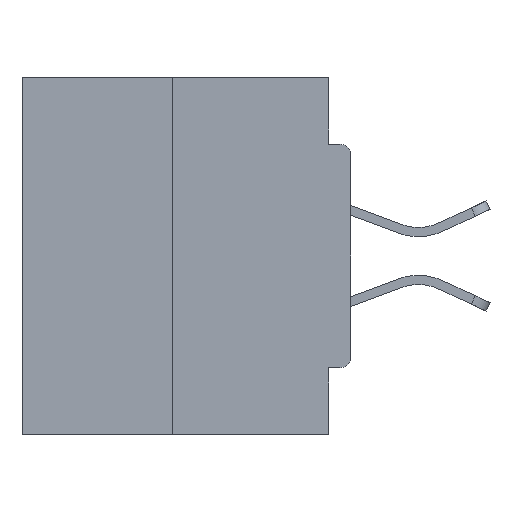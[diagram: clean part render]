
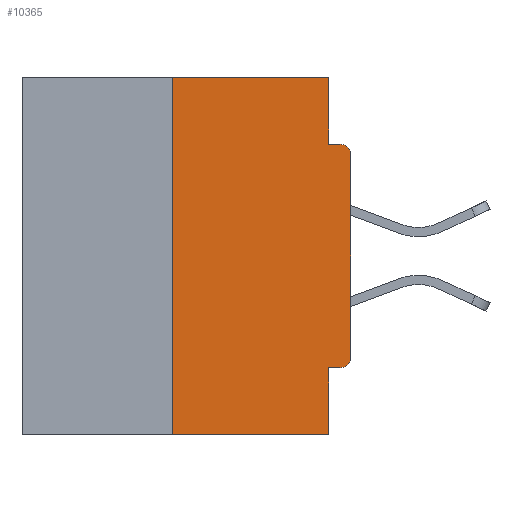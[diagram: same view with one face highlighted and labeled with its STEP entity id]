
A CAD part, left-side view. The second image highlights one B-rep face of the part: STEP entity #10365.
In plain terms, the highlighted planar face has unit normal (-1, 0, 0).
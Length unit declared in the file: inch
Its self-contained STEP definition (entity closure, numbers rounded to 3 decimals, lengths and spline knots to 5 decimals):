
#376 = VECTOR ( 'NONE', #6694, 39.37008 ) ;
#420 = CARTESIAN_POINT ( 'NONE',  ( 0., 0.031, -0.5 ) ) ;
#724 = CARTESIAN_POINT ( 'NONE',  ( 0., 0.031, 0. ) ) ;
#1459 = LINE ( 'NONE', #4553, #17671 ) ;
#1939 = AXIS2_PLACEMENT_3D ( 'NONE', #21516, #30189, #21997 ) ;
#2133 = ORIENTED_EDGE ( 'NONE', *, *, #30267, .T. ) ;
#2251 = EDGE_LOOP ( 'NONE', ( #25524, #4709, #2133, #23375, #24445, #21323, #34818, #24912, #11728, #12745 ) ) ;
#2271 = VECTOR ( 'NONE', #32624, 39.37008 ) ;
#2527 = LINE ( 'NONE', #28972, #376 ) ;
#2691 = LINE ( 'NONE', #9984, #2271 ) ;
#3945 = DIRECTION ( 'NONE',  ( 0., 0., -1. ) ) ;
#4428 = LINE ( 'NONE', #32149, #32079 ) ;
#4553 = CARTESIAN_POINT ( 'NONE',  ( 0., 0.46, 0. ) ) ;
#4709 = ORIENTED_EDGE ( 'NONE', *, *, #26231, .F. ) ;
#4724 = LINE ( 'NONE', #21037, #30146 ) ;
#4948 = PLANE ( 'NONE',  #1939 ) ;
#5551 = EDGE_CURVE ( 'NONE', #19096, #10292, #28142, .T. ) ;
#6506 = CARTESIAN_POINT ( 'NONE',  ( 0., 0.015, -0.4065 ) ) ;
#6694 = DIRECTION ( 'NONE',  ( 0., -1., 0. ) ) ;
#6846 = VERTEX_POINT ( 'NONE', #6506 ) ;
#8328 = VERTEX_POINT ( 'NONE', #724 ) ;
#9816 = CARTESIAN_POINT ( 'NONE',  ( 0., 0.031, -0.4065 ) ) ;
#9984 = CARTESIAN_POINT ( 'NONE',  ( 0., 0.031, -0.5 ) ) ;
#10292 = VERTEX_POINT ( 'NONE', #31576 ) ;
#10296 = CARTESIAN_POINT ( 'NONE',  ( 0., 0., -0.0935 ) ) ;
#10365 = ADVANCED_FACE ( 'NONE', ( #22548 ), #4948, .F. ) ;
#11728 = ORIENTED_EDGE ( 'NONE', *, *, #5551, .F. ) ;
#12745 = ORIENTED_EDGE ( 'NONE', *, *, #33685, .F. ) ;
#13715 = LINE ( 'NONE', #23313, #28602 ) ;
#13909 = VERTEX_POINT ( 'NONE', #420 ) ;
#14108 = CARTESIAN_POINT ( 'NONE',  ( 0., 0., -0.3915 ) ) ;
#15509 = CARTESIAN_POINT ( 'NONE',  ( 0., 0., -0.1085 ) ) ;
#15865 = VERTEX_POINT ( 'NONE', #9816 ) ;
#17099 = CIRCLE ( 'NONE', #17959, 0.015 ) ;
#17471 = CARTESIAN_POINT ( 'NONE',  ( 0., 0., -0.4065 ) ) ;
#17671 = VECTOR ( 'NONE', #32504, 39.37008 ) ;
#17777 = VERTEX_POINT ( 'NONE', #14108 ) ;
#17883 = CARTESIAN_POINT ( 'NONE',  ( 0., 0.25, 0. ) ) ;
#17959 = AXIS2_PLACEMENT_3D ( 'NONE', #34139, #26524, #26048 ) ;
#18327 = DIRECTION ( 'NONE',  ( 0., 0., 1. ) ) ;
#18349 = EDGE_CURVE ( 'NONE', #6846, #15865, #21427, .T. ) ;
#19096 = VERTEX_POINT ( 'NONE', #30796 ) ;
#19836 = VERTEX_POINT ( 'NONE', #20727 ) ;
#20727 = CARTESIAN_POINT ( 'NONE',  ( 0., 0.25, -0.5 ) ) ;
#20875 = CARTESIAN_POINT ( 'NONE',  ( 0., 0.015, -0.3915 ) ) ;
#21037 = CARTESIAN_POINT ( 'NONE',  ( 0., 0., 0. ) ) ;
#21323 = ORIENTED_EDGE ( 'NONE', *, *, #22582, .T. ) ;
#21427 = LINE ( 'NONE', #17471, #28906 ) ;
#21516 = CARTESIAN_POINT ( 'NONE',  ( 0., 0.46, 0. ) ) ;
#21997 = DIRECTION ( 'NONE',  ( 0., 0., -1. ) ) ;
#22548 = FACE_OUTER_BOUND ( 'NONE', #2251, .T. ) ;
#22582 = EDGE_CURVE ( 'NONE', #6846, #17777, #36241, .T. ) ;
#22743 = DIRECTION ( 'NONE',  ( 0., 1., 0. ) ) ;
#23313 = CARTESIAN_POINT ( 'NONE',  ( 0., 0.031, 0. ) ) ;
#23375 = ORIENTED_EDGE ( 'NONE', *, *, #35879, .F. ) ;
#24173 = DIRECTION ( 'NONE',  ( 0., 0., 1. ) ) ;
#24445 = ORIENTED_EDGE ( 'NONE', *, *, #18349, .F. ) ;
#24912 = ORIENTED_EDGE ( 'NONE', *, *, #34649, .T. ) ;
#25524 = ORIENTED_EDGE ( 'NONE', *, *, #33356, .F. ) ;
#25990 = VECTOR ( 'NONE', #35535, 39.37008 ) ;
#26048 = DIRECTION ( 'NONE',  ( 0., 0., -1. ) ) ;
#26112 = DIRECTION ( 'NONE',  ( 0., 0., -1. ) ) ;
#26231 = EDGE_CURVE ( 'NONE', #19836, #28730, #4428, .T. ) ;
#26524 = DIRECTION ( 'NONE',  ( -1., 0., 0. ) ) ;
#27965 = AXIS2_PLACEMENT_3D ( 'NONE', #20875, #32372, #3945 ) ;
#28142 = LINE ( 'NONE', #10296, #25990 ) ;
#28602 = VECTOR ( 'NONE', #26112, 39.37008 ) ;
#28730 = VERTEX_POINT ( 'NONE', #17883 ) ;
#28906 = VECTOR ( 'NONE', #22743, 39.37008 ) ;
#28972 = CARTESIAN_POINT ( 'NONE',  ( 0., 0.46, -0.5 ) ) ;
#29543 = EDGE_CURVE ( 'NONE', #17777, #29985, #4724, .T. ) ;
#29985 = VERTEX_POINT ( 'NONE', #15509 ) ;
#30146 = VECTOR ( 'NONE', #18327, 39.37008 ) ;
#30189 = DIRECTION ( 'NONE',  ( 1., 0., 0. ) ) ;
#30267 = EDGE_CURVE ( 'NONE', #19836, #13909, #2527, .T. ) ;
#30796 = CARTESIAN_POINT ( 'NONE',  ( 0., 0.031, -0.0935 ) ) ;
#31576 = CARTESIAN_POINT ( 'NONE',  ( 0., 0.015, -0.0935 ) ) ;
#32079 = VECTOR ( 'NONE', #24173, 39.37008 ) ;
#32149 = CARTESIAN_POINT ( 'NONE',  ( 0., 0.25, 0. ) ) ;
#32372 = DIRECTION ( 'NONE',  ( -1., 0., 0. ) ) ;
#32504 = DIRECTION ( 'NONE',  ( 0., -1., 0. ) ) ;
#32624 = DIRECTION ( 'NONE',  ( 0., 0., -1. ) ) ;
#33356 = EDGE_CURVE ( 'NONE', #28730, #8328, #1459, .T. ) ;
#33685 = EDGE_CURVE ( 'NONE', #8328, #19096, #13715, .T. ) ;
#34139 = CARTESIAN_POINT ( 'NONE',  ( 0., 0.015, -0.1085 ) ) ;
#34649 = EDGE_CURVE ( 'NONE', #29985, #10292, #17099, .T. ) ;
#34818 = ORIENTED_EDGE ( 'NONE', *, *, #29543, .T. ) ;
#35535 = DIRECTION ( 'NONE',  ( 0., -1., 0. ) ) ;
#35879 = EDGE_CURVE ( 'NONE', #15865, #13909, #2691, .T. ) ;
#36241 = CIRCLE ( 'NONE', #27965, 0.015 ) ;
